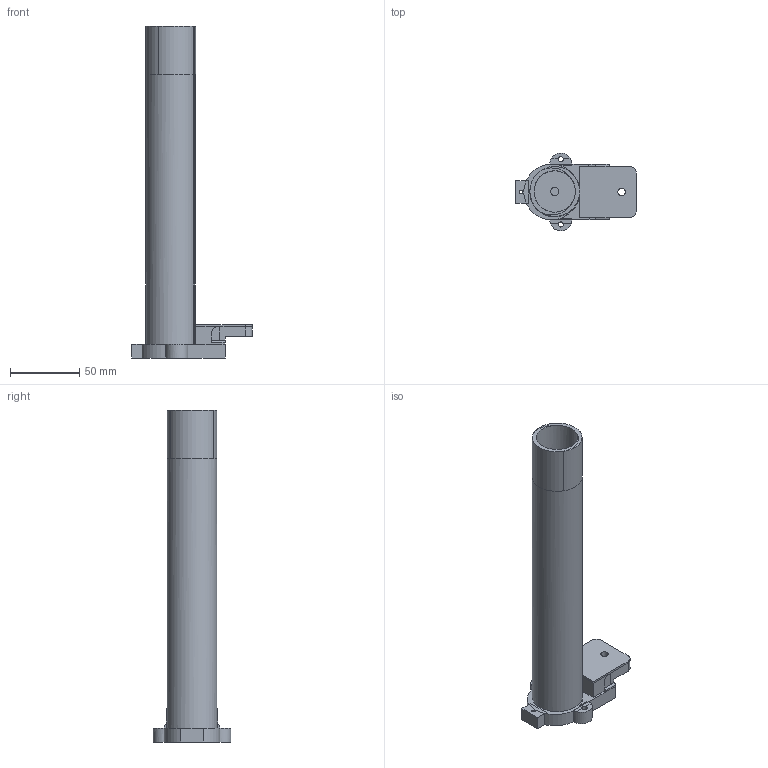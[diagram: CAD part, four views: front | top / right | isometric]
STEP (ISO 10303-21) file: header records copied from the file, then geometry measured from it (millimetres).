
FILE_DESCRIPTION(('FreeCAD Model'),'2;1');
FILE_NAME( 'ap9buffertube.step', '2017-11-13T22:53:44',('Author'),(''), 'Open CASCADE STEP processor 6.8','FreeCAD','Unknown');
FILE_SCHEMA(('AUTOMOTIVE_DESIGN_CC2 { 1 2 10303 214 -1 1 5 4 }'));
Length unit declared in the file: millimetre
Products named in the file (1): Pocket014
Bounding box: 86.94 x 56.2 x 240 mm (x, y, z)
Volume: 164463.6 mm3; surface area: 54960.4 mm2
Topology: 1 solids, 1 shells, 108 faces, 263 edges, 162 vertices
Faces by surface type: plane 75, cylinder 33
Full cylindrical faces by diameter (mm): 2.4 x1, 3.7 x2, 5.5 x3, 17.33 x1, 25 x1, 30 x2
Entity records: 6801 total; most frequent: CARTESIAN_POINT 1642, DIRECTION 961, ORIENTED_EDGE 526, PCURVE 526, DEFINITIONAL_REPRESENTATION 526, LINE 485, VECTOR 485, EDGE_CURVE 263
